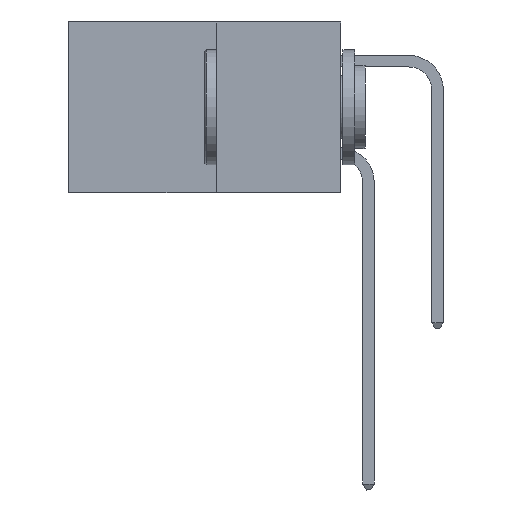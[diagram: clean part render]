
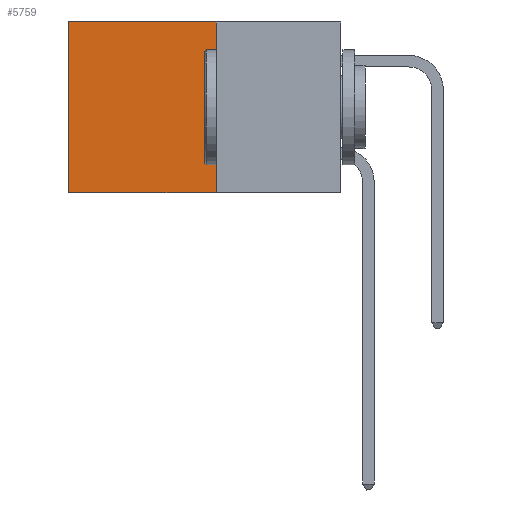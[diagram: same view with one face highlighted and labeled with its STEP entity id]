
A CAD part, left-side view. The second image highlights one B-rep face of the part: STEP entity #5759.
In plain terms, the highlighted planar face has unit normal (-1, 0, 0).
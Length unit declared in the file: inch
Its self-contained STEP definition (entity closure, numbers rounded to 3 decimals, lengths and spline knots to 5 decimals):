
#215 = VECTOR ( 'NONE', #5349, 39.37008 ) ;
#339 = EDGE_CURVE ( 'NONE', #11934, #9128, #11227, .T. ) ;
#370 = ORIENTED_EDGE ( 'NONE', *, *, #16393, .T. ) ;
#1347 = CARTESIAN_POINT ( 'NONE',  ( 0.277, 0.27, 0. ) ) ;
#1963 = PLANE ( 'NONE',  #16579 ) ;
#2227 = CARTESIAN_POINT ( 'NONE',  ( 0.277, 0.59, -0.37 ) ) ;
#2651 = CARTESIAN_POINT ( 'NONE',  ( 0.277, 0.27, 0. ) ) ;
#2866 = VECTOR ( 'NONE', #15725, 39.37008 ) ;
#3537 = VECTOR ( 'NONE', #10767, 39.37008 ) ;
#4019 = CARTESIAN_POINT ( 'NONE',  ( 0.277, 0.27, -0.37 ) ) ;
#4784 = DIRECTION ( 'NONE',  ( 1., 0., 0. ) ) ;
#4836 = VERTEX_POINT ( 'NONE', #5520 ) ;
#5186 = VERTEX_POINT ( 'NONE', #2227 ) ;
#5349 = DIRECTION ( 'NONE',  ( 0., 1., 0. ) ) ;
#5520 = CARTESIAN_POINT ( 'NONE',  ( 0.277, 0.59, 0. ) ) ;
#5540 = EDGE_CURVE ( 'NONE', #4836, #5186, #10375, .T. ) ;
#5759 = ADVANCED_FACE ( 'NONE', ( #10176 ), #1963, .F. ) ;
#7133 = LINE ( 'NONE', #4019, #215 ) ;
#7581 = EDGE_CURVE ( 'NONE', #9128, #5186, #7133, .T. ) ;
#8626 = EDGE_LOOP ( 'NONE', ( #9551, #9973, #14150, #370 ) ) ;
#9128 = VERTEX_POINT ( 'NONE', #11493 ) ;
#9551 = ORIENTED_EDGE ( 'NONE', *, *, #5540, .T. ) ;
#9973 = ORIENTED_EDGE ( 'NONE', *, *, #7581, .F. ) ;
#10176 = FACE_OUTER_BOUND ( 'NONE', #8626, .T. ) ;
#10375 = LINE ( 'NONE', #14481, #2866 ) ;
#10767 = DIRECTION ( 'NONE',  ( 0., 1., 0. ) ) ;
#11227 = LINE ( 'NONE', #14095, #14209 ) ;
#11305 = CARTESIAN_POINT ( 'NONE',  ( 0.277, 0.27, -0.37 ) ) ;
#11493 = CARTESIAN_POINT ( 'NONE',  ( 0.277, 0.27, -0.37 ) ) ;
#11523 = DIRECTION ( 'NONE',  ( 0., 0., -1. ) ) ;
#11934 = VERTEX_POINT ( 'NONE', #2651 ) ;
#13871 = DIRECTION ( 'NONE',  ( 0., 0., -1. ) ) ;
#14095 = CARTESIAN_POINT ( 'NONE',  ( 0.277, 0.27, -0.37 ) ) ;
#14150 = ORIENTED_EDGE ( 'NONE', *, *, #339, .F. ) ;
#14209 = VECTOR ( 'NONE', #11523, 39.37008 ) ;
#14481 = CARTESIAN_POINT ( 'NONE',  ( 0.277, 0.59, -0.37 ) ) ;
#15725 = DIRECTION ( 'NONE',  ( 0., 0., -1. ) ) ;
#16393 = EDGE_CURVE ( 'NONE', #11934, #4836, #16821, .T. ) ;
#16579 = AXIS2_PLACEMENT_3D ( 'NONE', #11305, #4784, #13871 ) ;
#16821 = LINE ( 'NONE', #1347, #3537 ) ;
